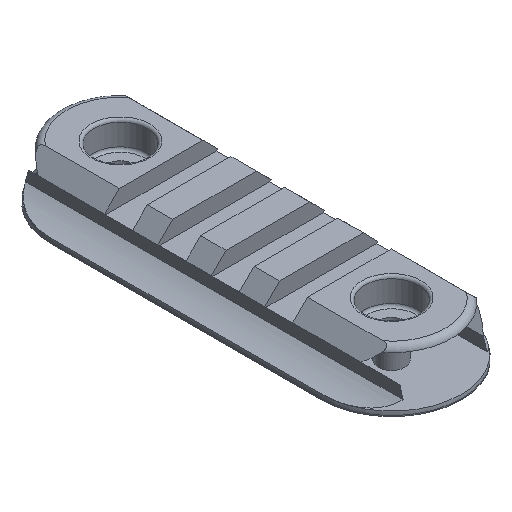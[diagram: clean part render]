
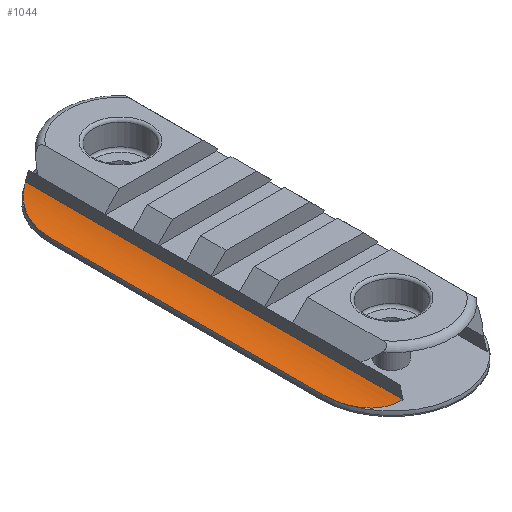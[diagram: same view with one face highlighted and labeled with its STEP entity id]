
A CAD part, isometric view. The second image highlights one B-rep face of the part: STEP entity #1044.
In plain terms, the highlighted cylindrical face has radius 9.838 mm (diameter 19.677 mm), a partial arc.
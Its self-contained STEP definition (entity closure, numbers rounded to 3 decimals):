
#27=B_SPLINE_CURVE_WITH_KNOTS('',3,(#1819,#1820,#1821,#1822,#1823,#1824,
#1825,#1826),.UNSPECIFIED.,.F.,.F.,(4,2,2,4),(4.044,4.359,
4.775,5.191),.UNSPECIFIED.);
#28=B_SPLINE_CURVE_WITH_KNOTS('',3,(#1838,#1839,#1840,#1841,#1842,#1843,
#1844,#1845,#1846,#1847,#1848,#1849),.UNSPECIFIED.,.F.,.F.,(4,2,2,2,2,4),
(1.162,1.413,1.665,1.916,2.167,
2.322),.UNSPECIFIED.);
#165=LINE('',#1835,#259);
#166=LINE('',#1850,#260);
#259=VECTOR('',#1423,10.);
#260=VECTOR('',#1426,10.);
#271=CYLINDRICAL_SURFACE('',#1155,9.838);
#319=FACE_OUTER_BOUND('',#379,.T.);
#379=EDGE_LOOP('',(#929,#930,#931,#932));
#497=VERTEX_POINT('',#1622);
#524=VERTEX_POINT('',#1815);
#525=VERTEX_POINT('',#1831);
#526=VERTEX_POINT('',#1837);
#664=EDGE_CURVE('',#524,#497,#27,.T.);
#667=EDGE_CURVE('',#525,#524,#165,.T.);
#668=EDGE_CURVE('',#526,#525,#28,.T.);
#669=EDGE_CURVE('',#497,#526,#166,.T.);
#929=ORIENTED_EDGE('',*,*,#664,.F.);
#930=ORIENTED_EDGE('',*,*,#667,.F.);
#931=ORIENTED_EDGE('',*,*,#668,.F.);
#932=ORIENTED_EDGE('',*,*,#669,.F.);
#1044=ADVANCED_FACE('',(#319),#271,.F.);
#1155=AXIS2_PLACEMENT_3D('',#1836,#1424,#1425);
#1423=DIRECTION('',(0.,-1.,0.));
#1424=DIRECTION('center_axis',(0.,-1.,0.));
#1425=DIRECTION('ref_axis',(0.536,0.,-0.844));
#1426=DIRECTION('',(0.,1.,0.));
#1622=CARTESIAN_POINT('',(-31.945,-64.77,0.847));
#1815=CARTESIAN_POINT('',(-26.769,-74.747,2.381));
#1819=CARTESIAN_POINT('Ctrl Pts',(-26.769,-74.747,2.381));
#1820=CARTESIAN_POINT('Ctrl Pts',(-27.594,-74.24,1.857));
#1821=CARTESIAN_POINT('Ctrl Pts',(-28.415,-73.533,1.514));
#1822=CARTESIAN_POINT('Ctrl Pts',(-29.971,-71.724,1.023));
#1823=CARTESIAN_POINT('Ctrl Pts',(-30.723,-70.434,0.923));
#1824=CARTESIAN_POINT('Ctrl Pts',(-31.71,-67.651,0.839));
#1825=CARTESIAN_POINT('Ctrl Pts',(-31.945,-66.158,0.847));
#1826=CARTESIAN_POINT('Ctrl Pts',(-31.945,-64.77,0.847));
#1831=CARTESIAN_POINT('',(-26.769,-3.993,2.381));
#1835=CARTESIAN_POINT('',(-26.769,0.,2.381));
#1836=CARTESIAN_POINT('Origin',(-32.046,0.,10.684));
#1837=CARTESIAN_POINT('',(-31.945,-13.97,0.847));
#1838=CARTESIAN_POINT('Ctrl Pts',(-31.945,-13.97,0.847));
#1839=CARTESIAN_POINT('Ctrl Pts',(-31.945,-13.133,0.847));
#1840=CARTESIAN_POINT('Ctrl Pts',(-31.863,-12.268,0.846));
#1841=CARTESIAN_POINT('Ctrl Pts',(-31.518,-10.56,0.859));
#1842=CARTESIAN_POINT('Ctrl Pts',(-31.255,-9.716,0.872));
#1843=CARTESIAN_POINT('Ctrl Pts',(-30.562,-8.117,0.952));
#1844=CARTESIAN_POINT('Ctrl Pts',(-30.13,-7.36,1.021));
#1845=CARTESIAN_POINT('Ctrl Pts',(-29.134,-5.994,1.273));
#1846=CARTESIAN_POINT('Ctrl Pts',(-28.57,-5.385,1.457));
#1847=CARTESIAN_POINT('Ctrl Pts',(-27.598,-4.552,1.899));
#1848=CARTESIAN_POINT('Ctrl Pts',(-27.186,-4.249,2.116));
#1849=CARTESIAN_POINT('Ctrl Pts',(-26.769,-3.993,2.381));
#1850=CARTESIAN_POINT('',(-31.945,-20.32,0.847));
